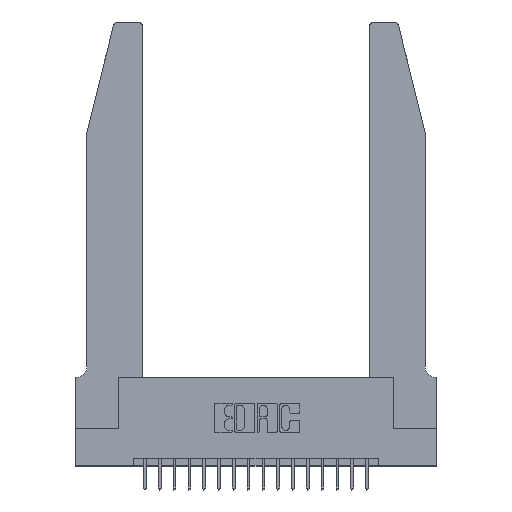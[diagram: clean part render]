
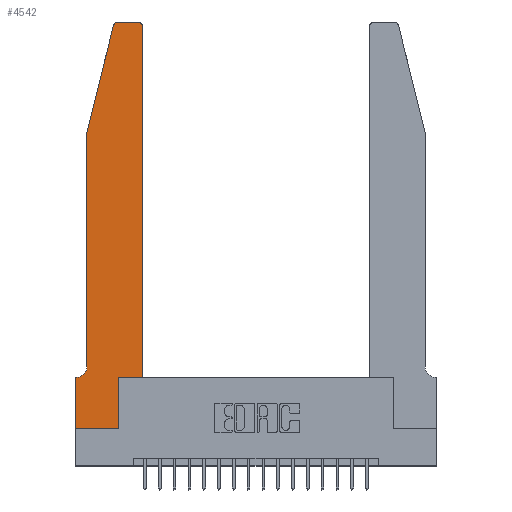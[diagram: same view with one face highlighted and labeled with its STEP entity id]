
A CAD part, top view. The second image highlights one B-rep face of the part: STEP entity #4542.
In plain terms, the highlighted planar face has unit normal (0, 0, 1).
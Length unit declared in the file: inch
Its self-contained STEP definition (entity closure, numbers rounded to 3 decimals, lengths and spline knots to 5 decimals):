
#114 = DIRECTION ( 'NONE',  ( 1., 0., 0. ) ) ;
#230 = EDGE_CURVE ( 'NONE', #2111, #11463, #18533, .T. ) ;
#477 = EDGE_CURVE ( 'NONE', #14817, #10681, #3397, .T. ) ;
#685 = FACE_OUTER_BOUND ( 'NONE', #6740, .T. ) ;
#746 = DIRECTION ( 'NONE',  ( 0., -1., 0. ) ) ;
#1190 = ORIENTED_EDGE ( 'NONE', *, *, #1574, .T. ) ;
#1428 = LINE ( 'NONE', #20608, #2672 ) ;
#1574 = EDGE_CURVE ( 'NONE', #14837, #7076, #8596, .T. ) ;
#1615 = DIRECTION ( 'NONE',  ( -1., 0., 0. ) ) ;
#1697 = VERTEX_POINT ( 'NONE', #15253 ) ;
#2005 = CARTESIAN_POINT ( 'NONE',  ( 0., 0.35, 0.37 ) ) ;
#2111 = VERTEX_POINT ( 'NONE', #3245 ) ;
#2202 = CARTESIAN_POINT ( 'NONE',  ( 0.2865, 0.35, 0.37 ) ) ;
#2672 = VECTOR ( 'NONE', #2981, 39.37008 ) ;
#2716 = EDGE_CURVE ( 'NONE', #3969, #8338, #3306, .T. ) ;
#2808 = EDGE_CURVE ( 'NONE', #8338, #6647, #11542, .T. ) ;
#2834 = EDGE_CURVE ( 'NONE', #6647, #1697, #14100, .T. ) ;
#2939 = CARTESIAN_POINT ( 'NONE',  ( 0.4505, 2.72, 0.37 ) ) ;
#2981 = DIRECTION ( 'NONE',  ( 1., 0., 0. ) ) ;
#3243 = EDGE_CURVE ( 'NONE', #12365, #14817, #5252, .T. ) ;
#3245 = CARTESIAN_POINT ( 'NONE',  ( 0.0755, 2., 0.37 ) ) ;
#3306 = CIRCLE ( 'NONE', #14866, 0.03 ) ;
#3397 = LINE ( 'NONE', #18416, #16741 ) ;
#3969 = VERTEX_POINT ( 'NONE', #2939 ) ;
#4357 = VECTOR ( 'NONE', #7074, 39.37008 ) ;
#4542 = ADVANCED_FACE ( 'NONE', ( #685 ), #11210, .T. ) ;
#5132 = VECTOR ( 'NONE', #7522, 39.37008 ) ;
#5248 = DIRECTION ( 'NONE',  ( -1., 0., 0. ) ) ;
#5252 = LINE ( 'NONE', #10208, #11023 ) ;
#6036 = CIRCLE ( 'NONE', #18827, 0.07 ) ;
#6050 = ORIENTED_EDGE ( 'NONE', *, *, #477, .T. ) ;
#6291 = EDGE_CURVE ( 'NONE', #10681, #14837, #9109, .T. ) ;
#6364 = VECTOR ( 'NONE', #19044, 39.37008 ) ;
#6414 = ORIENTED_EDGE ( 'NONE', *, *, #230, .T. ) ;
#6647 = VERTEX_POINT ( 'NONE', #11903 ) ;
#6740 = EDGE_LOOP ( 'NONE', ( #17311, #15695, #18859, #6414, #13579, #15163, #6050, #16874, #1190, #7485, #17515, #18062 ) ) ;
#7074 = DIRECTION ( 'NONE',  ( 0., 1., 0. ) ) ;
#7076 = VERTEX_POINT ( 'NONE', #10319 ) ;
#7253 = DIRECTION ( 'NONE',  ( 0., 0., -1. ) ) ;
#7301 = VECTOR ( 'NONE', #1615, 39.37008 ) ;
#7392 = DIRECTION ( 'NONE',  ( -0.239, -0.971, 0. ) ) ;
#7431 = CARTESIAN_POINT ( 'NONE',  ( 0.4205, 2.72, 0.37 ) ) ;
#7485 = ORIENTED_EDGE ( 'NONE', *, *, #20811, .T. ) ;
#7522 = DIRECTION ( 'NONE',  ( 0., -1., 0. ) ) ;
#7686 = DIRECTION ( 'NONE',  ( -1., 0., 0. ) ) ;
#7809 = CARTESIAN_POINT ( 'NONE',  ( 0., 0., 0.37 ) ) ;
#8338 = VERTEX_POINT ( 'NONE', #16389 ) ;
#8596 = LINE ( 'NONE', #2202, #4357 ) ;
#9109 = LINE ( 'NONE', #10798, #6364 ) ;
#9851 = DIRECTION ( 'NONE',  ( 0., 0., 1. ) ) ;
#10208 = CARTESIAN_POINT ( 'NONE',  ( 0.0755, 0.35, 0.37 ) ) ;
#10219 = VERTEX_POINT ( 'NONE', #12627 ) ;
#10319 = CARTESIAN_POINT ( 'NONE',  ( 0.2865, 0.35, 0.37 ) ) ;
#10530 = CARTESIAN_POINT ( 'NONE',  ( 0.0755, 0.42, 0.37 ) ) ;
#10681 = VERTEX_POINT ( 'NONE', #7809 ) ;
#10783 = CARTESIAN_POINT ( 'NONE',  ( 0.4505, 0.35, 0.37 ) ) ;
#10798 = CARTESIAN_POINT ( 'NONE',  ( 0., 0., 0.37 ) ) ;
#10899 = LINE ( 'NONE', #10783, #15468 ) ;
#11023 = VECTOR ( 'NONE', #5248, 39.37008 ) ;
#11210 = PLANE ( 'NONE',  #16812 ) ;
#11350 = EDGE_CURVE ( 'NONE', #10219, #3969, #10899, .T. ) ;
#11463 = VERTEX_POINT ( 'NONE', #10530 ) ;
#11542 = LINE ( 'NONE', #14662, #7301 ) ;
#11903 = CARTESIAN_POINT ( 'NONE',  ( 0.284, 2.75, 0.37 ) ) ;
#12365 = VERTEX_POINT ( 'NONE', #12884 ) ;
#12627 = CARTESIAN_POINT ( 'NONE',  ( 0.4505, 0.35, 0.37 ) ) ;
#12661 = DIRECTION ( 'NONE',  ( 1., 0., 0. ) ) ;
#12884 = CARTESIAN_POINT ( 'NONE',  ( 0.0055, 0.35, 0.37 ) ) ;
#13120 = DIRECTION ( 'NONE',  ( 1., 0., 0. ) ) ;
#13579 = ORIENTED_EDGE ( 'NONE', *, *, #13740, .T. ) ;
#13740 = EDGE_CURVE ( 'NONE', #11463, #12365, #6036, .T. ) ;
#13913 = DIRECTION ( 'NONE',  ( 0., 0., 1. ) ) ;
#13978 = LINE ( 'NONE', #18480, #14972 ) ;
#14100 = CIRCLE ( 'NONE', #19242, 0.03 ) ;
#14126 = DIRECTION ( 'NONE',  ( 0., 1., 0. ) ) ;
#14457 = DIRECTION ( 'NONE',  ( 0., 0., 1. ) ) ;
#14619 = CARTESIAN_POINT ( 'NONE',  ( 0., 0.35, 0.37 ) ) ;
#14662 = CARTESIAN_POINT ( 'NONE',  ( 0.2605, 2.75, 0.37 ) ) ;
#14817 = VERTEX_POINT ( 'NONE', #2005 ) ;
#14837 = VERTEX_POINT ( 'NONE', #17647 ) ;
#14866 = AXIS2_PLACEMENT_3D ( 'NONE', #7431, #13913, #12661 ) ;
#14972 = VECTOR ( 'NONE', #7392, 39.37008 ) ;
#15163 = ORIENTED_EDGE ( 'NONE', *, *, #3243, .T. ) ;
#15253 = CARTESIAN_POINT ( 'NONE',  ( 0.25487, 2.72718, 0.37 ) ) ;
#15468 = VECTOR ( 'NONE', #14126, 39.37008 ) ;
#15695 = ORIENTED_EDGE ( 'NONE', *, *, #2834, .T. ) ;
#16389 = CARTESIAN_POINT ( 'NONE',  ( 0.4205, 2.75, 0.37 ) ) ;
#16741 = VECTOR ( 'NONE', #746, 39.37008 ) ;
#16812 = AXIS2_PLACEMENT_3D ( 'NONE', #14619, #9851, #13120 ) ;
#16848 = EDGE_CURVE ( 'NONE', #1697, #2111, #13978, .T. ) ;
#16874 = ORIENTED_EDGE ( 'NONE', *, *, #6291, .T. ) ;
#16926 = CARTESIAN_POINT ( 'NONE',  ( 0.0055, 0.42, 0.37 ) ) ;
#17311 = ORIENTED_EDGE ( 'NONE', *, *, #2808, .T. ) ;
#17515 = ORIENTED_EDGE ( 'NONE', *, *, #11350, .T. ) ;
#17647 = CARTESIAN_POINT ( 'NONE',  ( 0.2865, 0., 0.37 ) ) ;
#17729 = CARTESIAN_POINT ( 'NONE',  ( 0.284, 2.72, 0.37 ) ) ;
#18062 = ORIENTED_EDGE ( 'NONE', *, *, #2716, .T. ) ;
#18416 = CARTESIAN_POINT ( 'NONE',  ( 0., 0., 0.37 ) ) ;
#18480 = CARTESIAN_POINT ( 'NONE',  ( 0.0755, 2., 0.37 ) ) ;
#18533 = LINE ( 'NONE', #18683, #5132 ) ;
#18683 = CARTESIAN_POINT ( 'NONE',  ( 0.0755, 2., 0.37 ) ) ;
#18827 = AXIS2_PLACEMENT_3D ( 'NONE', #16926, #7253, #7686 ) ;
#18859 = ORIENTED_EDGE ( 'NONE', *, *, #16848, .T. ) ;
#19044 = DIRECTION ( 'NONE',  ( 1., 0., 0. ) ) ;
#19242 = AXIS2_PLACEMENT_3D ( 'NONE', #17729, #14457, #114 ) ;
#20608 = CARTESIAN_POINT ( 'NONE',  ( 0.4505, 0.35, 0.37 ) ) ;
#20811 = EDGE_CURVE ( 'NONE', #7076, #10219, #1428, .T. ) ;
